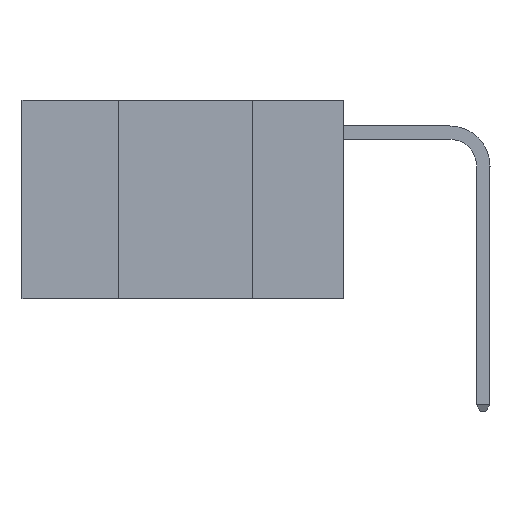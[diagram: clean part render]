
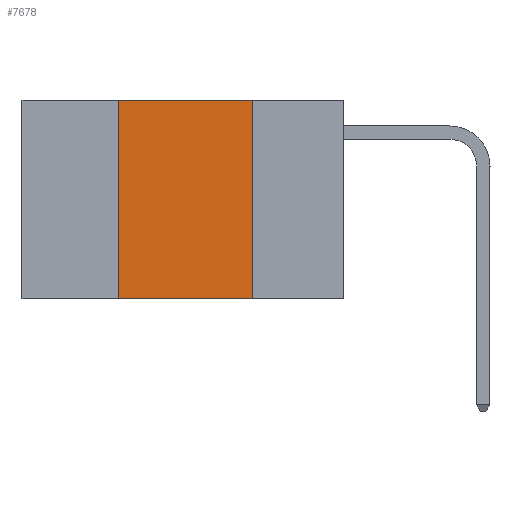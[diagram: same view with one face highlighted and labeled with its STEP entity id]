
A CAD part, left-side view. The second image highlights one B-rep face of the part: STEP entity #7678.
In plain terms, the highlighted planar face has unit normal (-1, 0, 0).
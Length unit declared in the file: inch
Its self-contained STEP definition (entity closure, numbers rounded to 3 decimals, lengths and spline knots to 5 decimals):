
#289 = VECTOR ( 'NONE', #6535, 39.37008 ) ;
#1202 = CARTESIAN_POINT ( 'NONE',  ( 0., 0.17, -0.37 ) ) ;
#1589 = VERTEX_POINT ( 'NONE', #6717 ) ;
#2233 = AXIS2_PLACEMENT_3D ( 'NONE', #12176, #6177, #13133 ) ;
#2293 = VERTEX_POINT ( 'NONE', #1202 ) ;
#2619 = LINE ( 'NONE', #11293, #10386 ) ;
#2775 = LINE ( 'NONE', #12545, #5207 ) ;
#3223 = DIRECTION ( 'NONE',  ( 0., 0., -1. ) ) ;
#3540 = CARTESIAN_POINT ( 'NONE',  ( 0., 0.42, 0. ) ) ;
#4059 = FACE_OUTER_BOUND ( 'NONE', #7637, .T. ) ;
#4379 = EDGE_CURVE ( 'NONE', #9624, #1589, #7959, .T. ) ;
#4678 = ORIENTED_EDGE ( 'NONE', *, *, #7097, .F. ) ;
#4999 = ORIENTED_EDGE ( 'NONE', *, *, #7259, .T. ) ;
#5110 = CARTESIAN_POINT ( 'NONE',  ( 0., 0.6, 0. ) ) ;
#5168 = PLANE ( 'NONE',  #2233 ) ;
#5207 = VECTOR ( 'NONE', #7586, 39.37008 ) ;
#5517 = CARTESIAN_POINT ( 'NONE',  ( 0., 0.42, 0. ) ) ;
#6177 = DIRECTION ( 'NONE',  ( 1., 0., 0. ) ) ;
#6371 = VERTEX_POINT ( 'NONE', #13079 ) ;
#6535 = DIRECTION ( 'NONE',  ( 0., 0., 1. ) ) ;
#6717 = CARTESIAN_POINT ( 'NONE',  ( 0., 0.17, 0. ) ) ;
#7097 = EDGE_CURVE ( 'NONE', #1589, #2293, #2619, .T. ) ;
#7235 = EDGE_CURVE ( 'NONE', #6371, #9624, #8505, .T. ) ;
#7259 = EDGE_CURVE ( 'NONE', #6371, #2293, #2775, .T. ) ;
#7371 = ORIENTED_EDGE ( 'NONE', *, *, #4379, .F. ) ;
#7586 = DIRECTION ( 'NONE',  ( 0., -1., 0. ) ) ;
#7637 = EDGE_LOOP ( 'NONE', ( #4678, #7371, #12653, #4999 ) ) ;
#7678 = ADVANCED_FACE ( 'NONE', ( #4059 ), #5168, .F. ) ;
#7959 = LINE ( 'NONE', #5110, #10300 ) ;
#8505 = LINE ( 'NONE', #5517, #289 ) ;
#9624 = VERTEX_POINT ( 'NONE', #3540 ) ;
#10155 = DIRECTION ( 'NONE',  ( 0., -1., 0. ) ) ;
#10300 = VECTOR ( 'NONE', #10155, 39.37008 ) ;
#10386 = VECTOR ( 'NONE', #3223, 39.37008 ) ;
#11293 = CARTESIAN_POINT ( 'NONE',  ( 0., 0.17, 0. ) ) ;
#12176 = CARTESIAN_POINT ( 'NONE',  ( 0., 0.6, 0. ) ) ;
#12545 = CARTESIAN_POINT ( 'NONE',  ( 0., 0.6, -0.37 ) ) ;
#12653 = ORIENTED_EDGE ( 'NONE', *, *, #7235, .F. ) ;
#13079 = CARTESIAN_POINT ( 'NONE',  ( 0., 0.42, -0.37 ) ) ;
#13133 = DIRECTION ( 'NONE',  ( 0., 0., -1. ) ) ;
